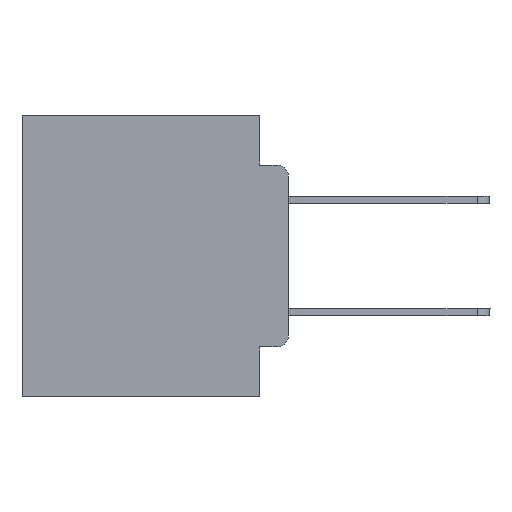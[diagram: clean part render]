
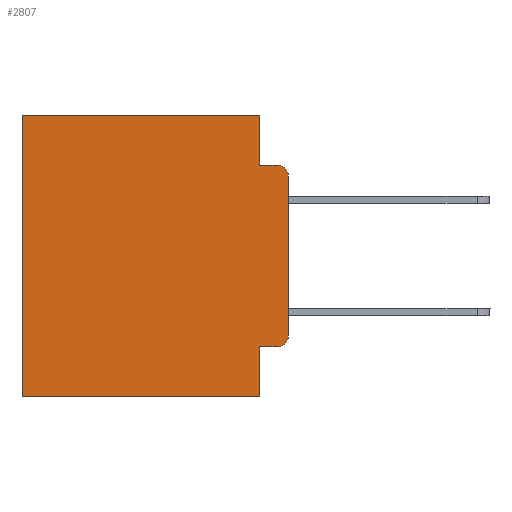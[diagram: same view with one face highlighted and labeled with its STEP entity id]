
A CAD part, left-side view. The second image highlights one B-rep face of the part: STEP entity #2807.
In plain terms, the highlighted planar face has unit normal (-1, 0, 0).
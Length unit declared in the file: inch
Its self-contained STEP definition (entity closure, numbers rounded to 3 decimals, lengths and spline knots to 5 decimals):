
#107 = VERTEX_POINT ( 'NONE', #10098 ) ;
#373 = DIRECTION ( 'NONE',  ( 0., 0., -1. ) ) ;
#829 = ORIENTED_EDGE ( 'NONE', *, *, #5194, .T. ) ;
#1266 = VERTEX_POINT ( 'NONE', #6430 ) ;
#1562 = DIRECTION ( 'NONE',  ( 0., 1., 0. ) ) ;
#2807 = ADVANCED_FACE ( 'NONE', ( #19655 ), #7604, .F. ) ;
#3295 = EDGE_CURVE ( 'NONE', #1266, #13498, #18663, .T. ) ;
#3357 = DIRECTION ( 'NONE',  ( 1., 0., 0. ) ) ;
#3905 = CARTESIAN_POINT ( 'NONE',  ( 0.298, 0.051, -0.0885 ) ) ;
#4388 = CARTESIAN_POINT ( 'NONE',  ( 0.298, 0., -0.5 ) ) ;
#4474 = AXIS2_PLACEMENT_3D ( 'NONE', #21255, #17321, #13188 ) ;
#4503 = DIRECTION ( 'NONE',  ( 0., 0., -1. ) ) ;
#4555 = ORIENTED_EDGE ( 'NONE', *, *, #21892, .F. ) ;
#4705 = VERTEX_POINT ( 'NONE', #3905 ) ;
#5069 = CIRCLE ( 'NONE', #8437, 0.02 ) ;
#5194 = EDGE_CURVE ( 'NONE', #24763, #5954, #6853, .T. ) ;
#5954 = VERTEX_POINT ( 'NONE', #6287 ) ;
#6170 = DIRECTION ( 'NONE',  ( 0., 0., -1. ) ) ;
#6287 = CARTESIAN_POINT ( 'NONE',  ( 0.298, 0.02, -0.4115 ) ) ;
#6423 = CARTESIAN_POINT ( 'NONE',  ( 0.298, 0., 0. ) ) ;
#6430 = CARTESIAN_POINT ( 'NONE',  ( 0.298, 0., -0.1085 ) ) ;
#6508 = ORIENTED_EDGE ( 'NONE', *, *, #3295, .T. ) ;
#6595 = ORIENTED_EDGE ( 'NONE', *, *, #14246, .T. ) ;
#6853 = LINE ( 'NONE', #23477, #12865 ) ;
#7430 = CARTESIAN_POINT ( 'NONE',  ( 0.298, 0., 0. ) ) ;
#7468 = VECTOR ( 'NONE', #1562, 39.37008 ) ;
#7604 = PLANE ( 'NONE',  #15826 ) ;
#7983 = ORIENTED_EDGE ( 'NONE', *, *, #16255, .F. ) ;
#8437 = AXIS2_PLACEMENT_3D ( 'NONE', #18499, #22513, #4503 ) ;
#8560 = ORIENTED_EDGE ( 'NONE', *, *, #17919, .T. ) ;
#9091 = LINE ( 'NONE', #7430, #7468 ) ;
#10098 = CARTESIAN_POINT ( 'NONE',  ( 0.298, 0.473, -0.5 ) ) ;
#10218 = EDGE_CURVE ( 'NONE', #24597, #4705, #16647, .T. ) ;
#11072 = CARTESIAN_POINT ( 'NONE',  ( 0.298, 0.051, 0. ) ) ;
#12510 = EDGE_CURVE ( 'NONE', #4705, #13498, #23867, .T. ) ;
#12859 = VECTOR ( 'NONE', #26032, 39.37008 ) ;
#12865 = VECTOR ( 'NONE', #22218, 39.37008 ) ;
#13188 = DIRECTION ( 'NONE',  ( 0., 0., -1. ) ) ;
#13498 = VERTEX_POINT ( 'NONE', #23040 ) ;
#14246 = EDGE_CURVE ( 'NONE', #22858, #107, #25989, .T. ) ;
#14304 = ORIENTED_EDGE ( 'NONE', *, *, #12510, .F. ) ;
#14503 = LINE ( 'NONE', #4388, #21765 ) ;
#15605 = VECTOR ( 'NONE', #20119, 39.37008 ) ;
#15826 = AXIS2_PLACEMENT_3D ( 'NONE', #25815, #3357, #21796 ) ;
#16255 = EDGE_CURVE ( 'NONE', #1266, #22205, #21989, .T. ) ;
#16647 = LINE ( 'NONE', #17904, #12859 ) ;
#17081 = ORIENTED_EDGE ( 'NONE', *, *, #19717, .F. ) ;
#17321 = DIRECTION ( 'NONE',  ( -1., 0., 0. ) ) ;
#17345 = CARTESIAN_POINT ( 'NONE',  ( 0.298, 0.051, -0.4115 ) ) ;
#17751 = ORIENTED_EDGE ( 'NONE', *, *, #20893, .T. ) ;
#17904 = CARTESIAN_POINT ( 'NONE',  ( 0.298, 0.051, 0. ) ) ;
#17919 = EDGE_CURVE ( 'NONE', #5954, #22205, #5069, .T. ) ;
#18499 = CARTESIAN_POINT ( 'NONE',  ( 0.298, 0.02, -0.3915 ) ) ;
#18641 = DIRECTION ( 'NONE',  ( 0., 1., 0. ) ) ;
#18663 = CIRCLE ( 'NONE', #4474, 0.02 ) ;
#19468 = EDGE_LOOP ( 'NONE', ( #7983, #6508, #14304, #25044, #17751, #6595, #4555, #17081, #829, #8560 ) ) ;
#19655 = FACE_OUTER_BOUND ( 'NONE', #19468, .T. ) ;
#19717 = EDGE_CURVE ( 'NONE', #24763, #22800, #25629, .T. ) ;
#19775 = CARTESIAN_POINT ( 'NONE',  ( 0.298, 0., -0.3915 ) ) ;
#20001 = CARTESIAN_POINT ( 'NONE',  ( 0.298, 0.473, 0. ) ) ;
#20119 = DIRECTION ( 'NONE',  ( 0., -1., 0. ) ) ;
#20893 = EDGE_CURVE ( 'NONE', #24597, #22858, #9091, .T. ) ;
#21201 = VECTOR ( 'NONE', #6170, 39.37008 ) ;
#21255 = CARTESIAN_POINT ( 'NONE',  ( 0.298, 0.02, -0.1085 ) ) ;
#21765 = VECTOR ( 'NONE', #18641, 39.37008 ) ;
#21796 = DIRECTION ( 'NONE',  ( 0., 0., -1. ) ) ;
#21866 = CARTESIAN_POINT ( 'NONE',  ( 0.298, 0.051, -0.5 ) ) ;
#21892 = EDGE_CURVE ( 'NONE', #22800, #107, #14503, .T. ) ;
#21989 = LINE ( 'NONE', #6423, #25802 ) ;
#22205 = VERTEX_POINT ( 'NONE', #19775 ) ;
#22218 = DIRECTION ( 'NONE',  ( 0., -1., 0. ) ) ;
#22438 = VECTOR ( 'NONE', #24457, 39.37008 ) ;
#22513 = DIRECTION ( 'NONE',  ( -1., 0., 0. ) ) ;
#22800 = VERTEX_POINT ( 'NONE', #21866 ) ;
#22858 = VERTEX_POINT ( 'NONE', #20001 ) ;
#23040 = CARTESIAN_POINT ( 'NONE',  ( 0.298, 0.02, -0.0885 ) ) ;
#23477 = CARTESIAN_POINT ( 'NONE',  ( 0.298, 0.051, -0.4115 ) ) ;
#23731 = CARTESIAN_POINT ( 'NONE',  ( 0.298, 0.473, 0. ) ) ;
#23867 = LINE ( 'NONE', #26102, #15605 ) ;
#24457 = DIRECTION ( 'NONE',  ( 0., 0., -1. ) ) ;
#24597 = VERTEX_POINT ( 'NONE', #11072 ) ;
#24640 = CARTESIAN_POINT ( 'NONE',  ( 0.298, 0.051, 0. ) ) ;
#24763 = VERTEX_POINT ( 'NONE', #17345 ) ;
#25044 = ORIENTED_EDGE ( 'NONE', *, *, #10218, .F. ) ;
#25629 = LINE ( 'NONE', #24640, #22438 ) ;
#25802 = VECTOR ( 'NONE', #373, 39.37008 ) ;
#25815 = CARTESIAN_POINT ( 'NONE',  ( 0.298, 0., 0. ) ) ;
#25989 = LINE ( 'NONE', #23731, #21201 ) ;
#26032 = DIRECTION ( 'NONE',  ( 0., 0., -1. ) ) ;
#26102 = CARTESIAN_POINT ( 'NONE',  ( 0.298, 0.051, -0.0885 ) ) ;
